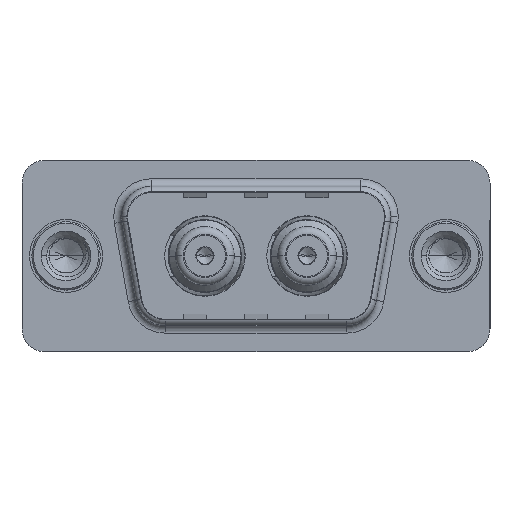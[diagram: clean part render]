
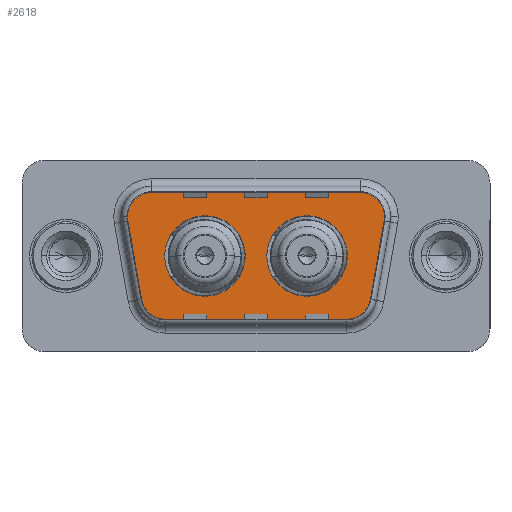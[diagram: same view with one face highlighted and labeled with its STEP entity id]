
A CAD part, top view. The second image highlights one B-rep face of the part: STEP entity #2618.
In plain terms, the highlighted planar face has unit normal (0, 0, 1).
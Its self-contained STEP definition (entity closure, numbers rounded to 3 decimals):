
#31 = DIRECTION ( 'NONE',  ( 0., 0., 1. ) ) ;
#570 = ORIENTED_EDGE ( 'NONE', *, *, #2992, .F. ) ;
#575 = CARTESIAN_POINT ( 'NONE',  ( 3.466, 2.553, 0. ) ) ;
#598 = CARTESIAN_POINT ( 'NONE',  ( 5.436, 2.9, 0. ) ) ;
#725 = DIRECTION ( 'NONE',  ( 0., 0., 1. ) ) ;
#764 = CARTESIAN_POINT ( 'NONE',  ( 6.49, 0., 0. ) ) ;
#781 = DIRECTION ( 'NONE',  ( 1., 0., 0. ) ) ;
#800 = CARTESIAN_POINT ( 'NONE',  ( 21.534, 2.553, 0. ) ) ;
#832 = CARTESIAN_POINT ( 'NONE',  ( 15.86, 0., 0. ) ) ;
#1104 = DIRECTION ( 'NONE',  ( 0.174, -0.985, 0. ) ) ;
#1254 = ORIENTED_EDGE ( 'NONE', *, *, #9317, .F. ) ;
#1270 = VERTEX_POINT ( 'NONE', #15748 ) ;
#1378 = CIRCLE ( 'NONE', #7811, 2.65 ) ;
#1510 = LINE ( 'NONE', #15989, #7692 ) ;
#1575 = EDGE_CURVE ( 'NONE', #2621, #15678, #2111, .T. ) ;
#1694 = ORIENTED_EDGE ( 'NONE', *, *, #5117, .T. ) ;
#2015 = DIRECTION ( 'NONE',  ( 1., 0., 0. ) ) ;
#2111 = LINE ( 'NONE', #6686, #15377 ) ;
#2172 = ORIENTED_EDGE ( 'NONE', *, *, #4841, .T. ) ;
#2302 = AXIS2_PLACEMENT_3D ( 'NONE', #6378, #15147, #7611 ) ;
#2562 = EDGE_CURVE ( 'NONE', #14052, #13975, #4022, .T. ) ;
#2587 = EDGE_LOOP ( 'NONE', ( #1254, #4935 ) ) ;
#2618 = ADVANCED_FACE ( 'NONE', ( #13182, #6933, #9819 ), #8517, .T. ) ;
#2621 = VERTEX_POINT ( 'NONE', #8411 ) ;
#2683 = CARTESIAN_POINT ( 'NONE',  ( 6.459, -4.9, 0. ) ) ;
#2992 = EDGE_CURVE ( 'NONE', #10043, #5095, #14749, .T. ) ;
#3298 = AXIS2_PLACEMENT_3D ( 'NONE', #6025, #14782, #7265 ) ;
#3441 = CARTESIAN_POINT ( 'NONE',  ( 18.541, -4.9, 0. ) ) ;
#3603 = CARTESIAN_POINT ( 'NONE',  ( 9.14, 0., 0. ) ) ;
#3619 = VERTEX_POINT ( 'NONE', #13819 ) ;
#3685 = EDGE_CURVE ( 'NONE', #6641, #3619, #5136, .T. ) ;
#4022 = CIRCLE ( 'NONE', #5108, 2. ) ;
#4490 = VECTOR ( 'NONE', #12775, 1000. ) ;
#4521 = AXIS2_PLACEMENT_3D ( 'NONE', #6048, #5936, #5878 ) ;
#4785 = CIRCLE ( 'NONE', #15932, 2. ) ;
#4835 = DIRECTION ( 'NONE',  ( 1., 0., 0. ) ) ;
#4841 = EDGE_CURVE ( 'NONE', #1270, #6641, #10534, .T. ) ;
#4862 = ORIENTED_EDGE ( 'NONE', *, *, #15063, .T. ) ;
#4935 = ORIENTED_EDGE ( 'NONE', *, *, #12222, .F. ) ;
#5095 = VERTEX_POINT ( 'NONE', #6967 ) ;
#5108 = AXIS2_PLACEMENT_3D ( 'NONE', #10397, #10444, #15925 ) ;
#5117 = EDGE_CURVE ( 'NONE', #15678, #7740, #10540, .T. ) ;
#5136 = CIRCLE ( 'NONE', #12237, 2. ) ;
#5237 = ORIENTED_EDGE ( 'NONE', *, *, #1575, .T. ) ;
#5878 = DIRECTION ( 'NONE',  ( 1., 0., 0. ) ) ;
#5936 = DIRECTION ( 'NONE',  ( 0., 0., 1. ) ) ;
#5960 = CARTESIAN_POINT ( 'NONE',  ( 19.564, 2.9, 0. ) ) ;
#6025 = CARTESIAN_POINT ( 'NONE',  ( 18.541, -2.9, 0. ) ) ;
#6029 = VERTEX_POINT ( 'NONE', #11236 ) ;
#6048 = CARTESIAN_POINT ( 'NONE',  ( 9.14, 0., 0. ) ) ;
#6110 = CARTESIAN_POINT ( 'NONE',  ( 13.21, 0., 0. ) ) ;
#6222 = AXIS2_PLACEMENT_3D ( 'NONE', #832, #9439, #2015 ) ;
#6378 = CARTESIAN_POINT ( 'NONE',  ( 15.86, 0., 0. ) ) ;
#6641 = VERTEX_POINT ( 'NONE', #8600 ) ;
#6686 = CARTESIAN_POINT ( 'NONE',  ( 5.436, 4.9, 0. ) ) ;
#6933 = FACE_BOUND ( 'NONE', #13567, .T. ) ;
#6967 = CARTESIAN_POINT ( 'NONE',  ( 11.79, 0., 0. ) ) ;
#7162 = DIRECTION ( 'NONE',  ( 1., 0., 0. ) ) ;
#7210 = DIRECTION ( 'NONE',  ( -1., 0., 0. ) ) ;
#7229 = VECTOR ( 'NONE', #14584, 1000. ) ;
#7265 = DIRECTION ( 'NONE',  ( 1., 0., 0. ) ) ;
#7337 = CARTESIAN_POINT ( 'NONE',  ( 19.564, 2.9, 0. ) ) ;
#7611 = DIRECTION ( 'NONE',  ( 1., 0., 0. ) ) ;
#7692 = VECTOR ( 'NONE', #1104, 1000. ) ;
#7740 = VERTEX_POINT ( 'NONE', #575 ) ;
#7811 = AXIS2_PLACEMENT_3D ( 'NONE', #3603, #12300, #4835 ) ;
#8411 = CARTESIAN_POINT ( 'NONE',  ( 19.564, 4.9, 0. ) ) ;
#8517 = PLANE ( 'NONE',  #10936 ) ;
#8576 = DIRECTION ( 'NONE',  ( -1., 0., 0. ) ) ;
#8600 = CARTESIAN_POINT ( 'NONE',  ( 21.534, 2.553, 0. ) ) ;
#8931 = EDGE_CURVE ( 'NONE', #5095, #10043, #1378, .T. ) ;
#9003 = ORIENTED_EDGE ( 'NONE', *, *, #2562, .T. ) ;
#9317 = EDGE_CURVE ( 'NONE', #6029, #9535, #12082, .T. ) ;
#9439 = DIRECTION ( 'NONE',  ( 0., 0., 1. ) ) ;
#9535 = VERTEX_POINT ( 'NONE', #6110 ) ;
#9797 = EDGE_CURVE ( 'NONE', #13975, #15592, #11068, .T. ) ;
#9819 = FACE_OUTER_BOUND ( 'NONE', #12193, .T. ) ;
#10043 = VERTEX_POINT ( 'NONE', #764 ) ;
#10207 = CIRCLE ( 'NONE', #2302, 2.65 ) ;
#10397 = CARTESIAN_POINT ( 'NONE',  ( 6.459, -2.9, 0. ) ) ;
#10444 = DIRECTION ( 'NONE',  ( 0., 0., 1. ) ) ;
#10534 = LINE ( 'NONE', #800, #7229 ) ;
#10540 = CIRCLE ( 'NONE', #14061, 2. ) ;
#10936 = AXIS2_PLACEMENT_3D ( 'NONE', #14071, #725, #781 ) ;
#11068 = LINE ( 'NONE', #15255, #4490 ) ;
#11161 = ORIENTED_EDGE ( 'NONE', *, *, #3685, .T. ) ;
#11236 = CARTESIAN_POINT ( 'NONE',  ( 18.51, 0., 0. ) ) ;
#11587 = CARTESIAN_POINT ( 'NONE',  ( 4.489, -3.247, 0. ) ) ;
#11635 = ORIENTED_EDGE ( 'NONE', *, *, #8931, .F. ) ;
#11663 = DIRECTION ( 'NONE',  ( 0., 0., 1. ) ) ;
#12082 = CIRCLE ( 'NONE', #6222, 2.65 ) ;
#12193 = EDGE_LOOP ( 'NONE', ( #14976, #2172, #11161, #15844, #5237, #1694, #4862, #9003, #13181 ) ) ;
#12222 = EDGE_CURVE ( 'NONE', #9535, #6029, #10207, .T. ) ;
#12237 = AXIS2_PLACEMENT_3D ( 'NONE', #5960, #13096, #13493 ) ;
#12300 = DIRECTION ( 'NONE',  ( 0., 0., 1. ) ) ;
#12775 = DIRECTION ( 'NONE',  ( 1., 0., 0. ) ) ;
#13096 = DIRECTION ( 'NONE',  ( 0., 0., 1. ) ) ;
#13171 = CIRCLE ( 'NONE', #3298, 2. ) ;
#13181 = ORIENTED_EDGE ( 'NONE', *, *, #9797, .T. ) ;
#13182 = FACE_BOUND ( 'NONE', #2587, .T. ) ;
#13493 = DIRECTION ( 'NONE',  ( -1., 0., 0. ) ) ;
#13562 = CARTESIAN_POINT ( 'NONE',  ( 5.436, 4.9, 0. ) ) ;
#13567 = EDGE_LOOP ( 'NONE', ( #11635, #570 ) ) ;
#13819 = CARTESIAN_POINT ( 'NONE',  ( 21.564, 2.9, 0. ) ) ;
#13975 = VERTEX_POINT ( 'NONE', #2683 ) ;
#14052 = VERTEX_POINT ( 'NONE', #11587 ) ;
#14061 = AXIS2_PLACEMENT_3D ( 'NONE', #598, #11663, #7162 ) ;
#14071 = CARTESIAN_POINT ( 'NONE',  ( 18.541, -2.9, 0. ) ) ;
#14584 = DIRECTION ( 'NONE',  ( 0.174, 0.985, 0. ) ) ;
#14749 = CIRCLE ( 'NONE', #4521, 2.65 ) ;
#14782 = DIRECTION ( 'NONE',  ( 0., 0., 1. ) ) ;
#14976 = ORIENTED_EDGE ( 'NONE', *, *, #15638, .T. ) ;
#15063 = EDGE_CURVE ( 'NONE', #7740, #14052, #1510, .T. ) ;
#15119 = EDGE_CURVE ( 'NONE', #3619, #2621, #4785, .T. ) ;
#15147 = DIRECTION ( 'NONE',  ( 0., 0., 1. ) ) ;
#15255 = CARTESIAN_POINT ( 'NONE',  ( 6.459, -4.9, 0. ) ) ;
#15377 = VECTOR ( 'NONE', #7210, 1000. ) ;
#15592 = VERTEX_POINT ( 'NONE', #3441 ) ;
#15638 = EDGE_CURVE ( 'NONE', #15592, #1270, #13171, .T. ) ;
#15678 = VERTEX_POINT ( 'NONE', #13562 ) ;
#15748 = CARTESIAN_POINT ( 'NONE',  ( 20.511, -3.247, 0. ) ) ;
#15844 = ORIENTED_EDGE ( 'NONE', *, *, #15119, .T. ) ;
#15925 = DIRECTION ( 'NONE',  ( -1., 0., 0. ) ) ;
#15932 = AXIS2_PLACEMENT_3D ( 'NONE', #7337, #31, #8576 ) ;
#15989 = CARTESIAN_POINT ( 'NONE',  ( 3.466, 2.553, 0. ) ) ;
